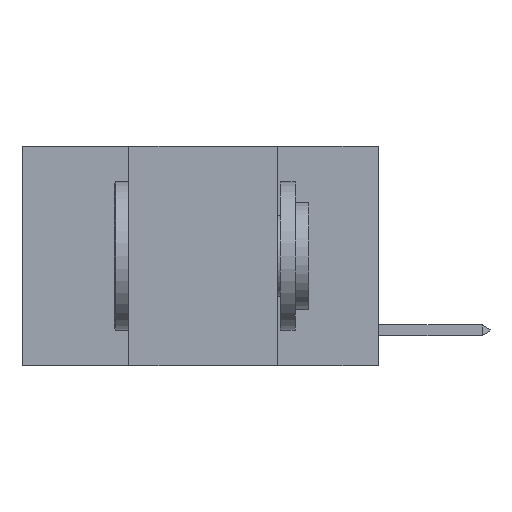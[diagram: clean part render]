
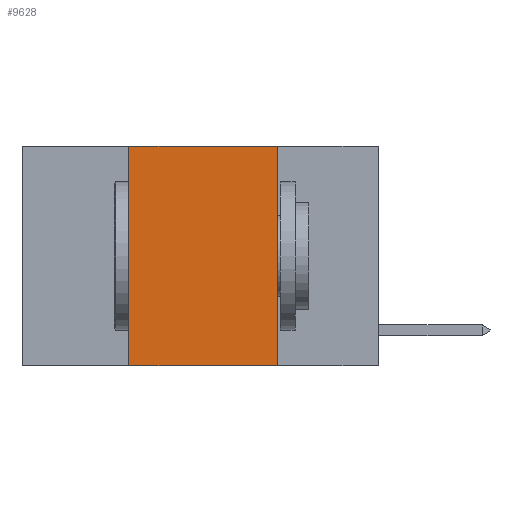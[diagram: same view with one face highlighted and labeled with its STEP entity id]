
A CAD part, left-side view. The second image highlights one B-rep face of the part: STEP entity #9628.
In plain terms, the highlighted planar face has unit normal (-1, 0, 0).
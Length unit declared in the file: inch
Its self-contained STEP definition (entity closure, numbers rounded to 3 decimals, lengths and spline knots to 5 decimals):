
#82 = AXIS2_PLACEMENT_3D ( 'NONE', #6454, #10893, #7868 ) ;
#95 = CARTESIAN_POINT ( 'NONE',  ( 0., 0.6, -0.37 ) ) ;
#469 = CARTESIAN_POINT ( 'NONE',  ( 0., 0.42, -0.37 ) ) ;
#587 = CARTESIAN_POINT ( 'NONE',  ( 0., 0.17, 0. ) ) ;
#695 = EDGE_CURVE ( 'NONE', #5703, #5861, #6214, .T. ) ;
#781 = LINE ( 'NONE', #95, #2300 ) ;
#937 = VECTOR ( 'NONE', #2406, 39.37008 ) ;
#1180 = PLANE ( 'NONE',  #82 ) ;
#1229 = VERTEX_POINT ( 'NONE', #5430 ) ;
#1489 = CARTESIAN_POINT ( 'NONE',  ( 0., 0.42, 0. ) ) ;
#2029 = FACE_OUTER_BOUND ( 'NONE', #2128, .T. ) ;
#2128 = EDGE_LOOP ( 'NONE', ( #7596, #11028, #4476, #2748 ) ) ;
#2300 = VECTOR ( 'NONE', #2604, 39.37008 ) ;
#2406 = DIRECTION ( 'NONE',  ( 0., 0., -1. ) ) ;
#2604 = DIRECTION ( 'NONE',  ( 0., -1., 0. ) ) ;
#2707 = EDGE_CURVE ( 'NONE', #5861, #6402, #3127, .T. ) ;
#2748 = ORIENTED_EDGE ( 'NONE', *, *, #7704, .T. ) ;
#3127 = LINE ( 'NONE', #9362, #8605 ) ;
#3519 = CARTESIAN_POINT ( 'NONE',  ( 0., 0.17, 0. ) ) ;
#3865 = EDGE_CURVE ( 'NONE', #6402, #1229, #8469, .T. ) ;
#4476 = ORIENTED_EDGE ( 'NONE', *, *, #695, .F. ) ;
#5430 = CARTESIAN_POINT ( 'NONE',  ( 0., 0.17, -0.37 ) ) ;
#5599 = DIRECTION ( 'NONE',  ( 0., -1., 0. ) ) ;
#5703 = VERTEX_POINT ( 'NONE', #469 ) ;
#5861 = VERTEX_POINT ( 'NONE', #1489 ) ;
#6214 = LINE ( 'NONE', #10604, #9691 ) ;
#6402 = VERTEX_POINT ( 'NONE', #3519 ) ;
#6454 = CARTESIAN_POINT ( 'NONE',  ( 0., 0.6, 0. ) ) ;
#7596 = ORIENTED_EDGE ( 'NONE', *, *, #3865, .F. ) ;
#7704 = EDGE_CURVE ( 'NONE', #5703, #1229, #781, .T. ) ;
#7868 = DIRECTION ( 'NONE',  ( 0., 0., -1. ) ) ;
#8469 = LINE ( 'NONE', #587, #937 ) ;
#8605 = VECTOR ( 'NONE', #5599, 39.37008 ) ;
#9362 = CARTESIAN_POINT ( 'NONE',  ( 0., 0.6, 0. ) ) ;
#9628 = ADVANCED_FACE ( 'NONE', ( #2029 ), #1180, .F. ) ;
#9691 = VECTOR ( 'NONE', #10929, 39.37008 ) ;
#10604 = CARTESIAN_POINT ( 'NONE',  ( 0., 0.42, 0. ) ) ;
#10893 = DIRECTION ( 'NONE',  ( 1., 0., 0. ) ) ;
#10929 = DIRECTION ( 'NONE',  ( 0., 0., 1. ) ) ;
#11028 = ORIENTED_EDGE ( 'NONE', *, *, #2707, .F. ) ;
